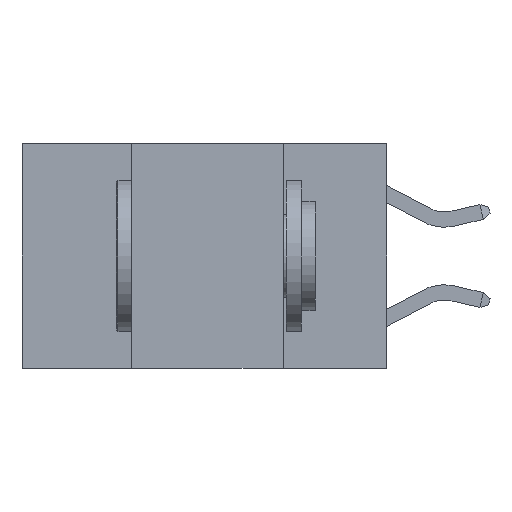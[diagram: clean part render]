
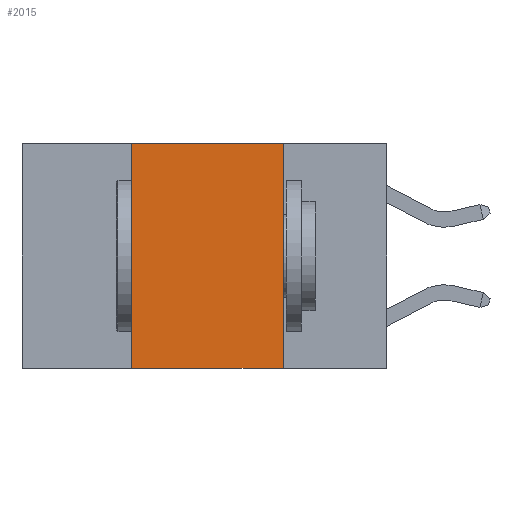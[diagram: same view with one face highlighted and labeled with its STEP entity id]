
A CAD part, left-side view. The second image highlights one B-rep face of the part: STEP entity #2015.
In plain terms, the highlighted planar face has unit normal (-1, 0, 0).
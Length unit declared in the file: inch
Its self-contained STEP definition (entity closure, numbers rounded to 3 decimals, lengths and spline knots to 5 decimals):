
#403 = VECTOR ( 'NONE', #3081, 39.37008 ) ;
#548 = LINE ( 'NONE', #12453, #5932 ) ;
#972 = VECTOR ( 'NONE', #7772, 39.37008 ) ;
#1569 = EDGE_LOOP ( 'NONE', ( #12603, #7224, #1858, #13267 ) ) ;
#1858 = ORIENTED_EDGE ( 'NONE', *, *, #12769, .F. ) ;
#2015 = ADVANCED_FACE ( 'NONE', ( #12632 ), #9433, .F. ) ;
#3081 = DIRECTION ( 'NONE',  ( 0., -1., 0. ) ) ;
#3754 = AXIS2_PLACEMENT_3D ( 'NONE', #11660, #11584, #11507 ) ;
#3838 = LINE ( 'NONE', #13119, #972 ) ;
#5270 = CARTESIAN_POINT ( 'NONE',  ( 0., 0.6, 0. ) ) ;
#5441 = EDGE_CURVE ( 'NONE', #6144, #13182, #8650, .T. ) ;
#5668 = CARTESIAN_POINT ( 'NONE',  ( 0., 0.6, -0.37 ) ) ;
#5750 = CARTESIAN_POINT ( 'NONE',  ( 0., 0.17, -0.37 ) ) ;
#5932 = VECTOR ( 'NONE', #11425, 39.37008 ) ;
#6119 = VERTEX_POINT ( 'NONE', #10611 ) ;
#6144 = VERTEX_POINT ( 'NONE', #12749 ) ;
#6434 = VERTEX_POINT ( 'NONE', #5750 ) ;
#7224 = ORIENTED_EDGE ( 'NONE', *, *, #5441, .F. ) ;
#7256 = EDGE_CURVE ( 'NONE', #13182, #6434, #548, .T. ) ;
#7390 = CARTESIAN_POINT ( 'NONE',  ( 0., 0.17, 0. ) ) ;
#7772 = DIRECTION ( 'NONE',  ( 0., 0., 1. ) ) ;
#8650 = LINE ( 'NONE', #5270, #403 ) ;
#9208 = VECTOR ( 'NONE', #11032, 39.37008 ) ;
#9433 = PLANE ( 'NONE',  #3754 ) ;
#10611 = CARTESIAN_POINT ( 'NONE',  ( 0., 0.42, -0.37 ) ) ;
#11032 = DIRECTION ( 'NONE',  ( 0., -1., 0. ) ) ;
#11425 = DIRECTION ( 'NONE',  ( 0., 0., -1. ) ) ;
#11507 = DIRECTION ( 'NONE',  ( 0., 0., -1. ) ) ;
#11584 = DIRECTION ( 'NONE',  ( 1., 0., 0. ) ) ;
#11660 = CARTESIAN_POINT ( 'NONE',  ( 0., 0.6, 0. ) ) ;
#12062 = LINE ( 'NONE', #5668, #9208 ) ;
#12453 = CARTESIAN_POINT ( 'NONE',  ( 0., 0.17, 0. ) ) ;
#12603 = ORIENTED_EDGE ( 'NONE', *, *, #7256, .F. ) ;
#12632 = FACE_OUTER_BOUND ( 'NONE', #1569, .T. ) ;
#12749 = CARTESIAN_POINT ( 'NONE',  ( 0., 0.42, 0. ) ) ;
#12769 = EDGE_CURVE ( 'NONE', #6119, #6144, #3838, .T. ) ;
#12787 = EDGE_CURVE ( 'NONE', #6119, #6434, #12062, .T. ) ;
#13119 = CARTESIAN_POINT ( 'NONE',  ( 0., 0.42, 0. ) ) ;
#13182 = VERTEX_POINT ( 'NONE', #7390 ) ;
#13267 = ORIENTED_EDGE ( 'NONE', *, *, #12787, .T. ) ;
